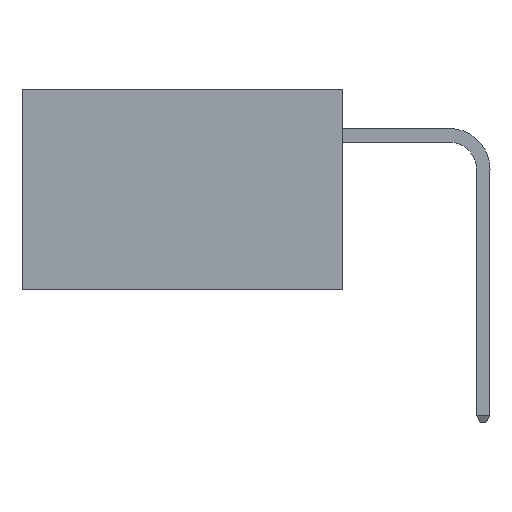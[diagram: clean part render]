
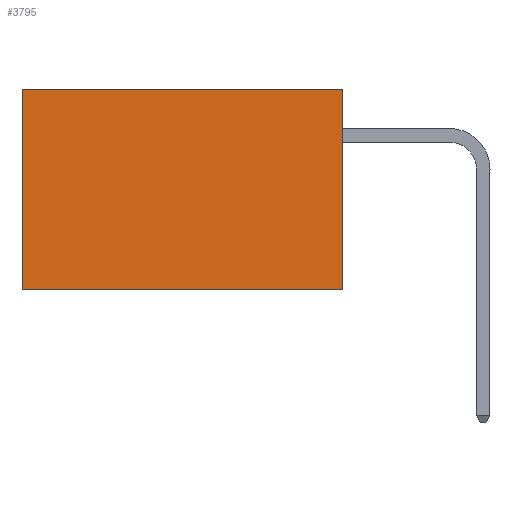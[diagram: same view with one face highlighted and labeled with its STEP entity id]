
A CAD part, left-side view. The second image highlights one B-rep face of the part: STEP entity #3795.
In plain terms, the highlighted planar face has unit normal (-1, 0, 0).
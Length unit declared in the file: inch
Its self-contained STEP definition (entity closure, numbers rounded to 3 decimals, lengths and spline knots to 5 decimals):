
#146 = VECTOR ( 'NONE', #2674, 39.37008 ) ;
#361 = EDGE_CURVE ( 'NONE', #4779, #3338, #7185, .T. ) ;
#392 = EDGE_CURVE ( 'NONE', #2401, #4779, #6876, .T. ) ;
#466 = VERTEX_POINT ( 'NONE', #5776 ) ;
#700 = CARTESIAN_POINT ( 'NONE',  ( 0.277, 0.59, -0.37 ) ) ;
#1150 = CARTESIAN_POINT ( 'NONE',  ( 0.277, 0., 0. ) ) ;
#1237 = EDGE_CURVE ( 'NONE', #466, #3338, #1565, .T. ) ;
#1284 = ORIENTED_EDGE ( 'NONE', *, *, #392, .F. ) ;
#1565 = LINE ( 'NONE', #700, #4852 ) ;
#1581 = EDGE_CURVE ( 'NONE', #2401, #466, #6718, .T. ) ;
#1897 = CARTESIAN_POINT ( 'NONE',  ( 0.277, 0., -0.37 ) ) ;
#2179 = CARTESIAN_POINT ( 'NONE',  ( 0.277, 0., 0. ) ) ;
#2296 = VECTOR ( 'NONE', #5864, 39.37008 ) ;
#2401 = VERTEX_POINT ( 'NONE', #2179 ) ;
#2417 = FACE_OUTER_BOUND ( 'NONE', #6230, .T. ) ;
#2646 = ORIENTED_EDGE ( 'NONE', *, *, #1237, .T. ) ;
#2674 = DIRECTION ( 'NONE',  ( 0., 1., 0. ) ) ;
#2972 = ORIENTED_EDGE ( 'NONE', *, *, #1581, .T. ) ;
#3303 = CARTESIAN_POINT ( 'NONE',  ( 0.277, 0., -0.37 ) ) ;
#3338 = VERTEX_POINT ( 'NONE', #6269 ) ;
#3795 = ADVANCED_FACE ( 'NONE', ( #2417 ), #6123, .F. ) ;
#3920 = DIRECTION ( 'NONE',  ( 0., 0., -1. ) ) ;
#4779 = VERTEX_POINT ( 'NONE', #3303 ) ;
#4852 = VECTOR ( 'NONE', #3920, 39.37008 ) ;
#5240 = ORIENTED_EDGE ( 'NONE', *, *, #361, .F. ) ;
#5384 = AXIS2_PLACEMENT_3D ( 'NONE', #6167, #6103, #6092 ) ;
#5776 = CARTESIAN_POINT ( 'NONE',  ( 0.277, 0.59, 0. ) ) ;
#5864 = DIRECTION ( 'NONE',  ( 0., 0., -1. ) ) ;
#6092 = DIRECTION ( 'NONE',  ( 0., 0., -1. ) ) ;
#6103 = DIRECTION ( 'NONE',  ( 1., 0., 0. ) ) ;
#6123 = PLANE ( 'NONE',  #5384 ) ;
#6167 = CARTESIAN_POINT ( 'NONE',  ( 0.277, 0., -0.37 ) ) ;
#6230 = EDGE_LOOP ( 'NONE', ( #2646, #5240, #1284, #2972 ) ) ;
#6269 = CARTESIAN_POINT ( 'NONE',  ( 0.277, 0.59, -0.37 ) ) ;
#6692 = CARTESIAN_POINT ( 'NONE',  ( 0.277, 0., -0.37 ) ) ;
#6718 = LINE ( 'NONE', #1150, #146 ) ;
#6876 = LINE ( 'NONE', #1897, #2296 ) ;
#7038 = VECTOR ( 'NONE', #7211, 39.37008 ) ;
#7185 = LINE ( 'NONE', #6692, #7038 ) ;
#7211 = DIRECTION ( 'NONE',  ( 0., 1., 0. ) ) ;
